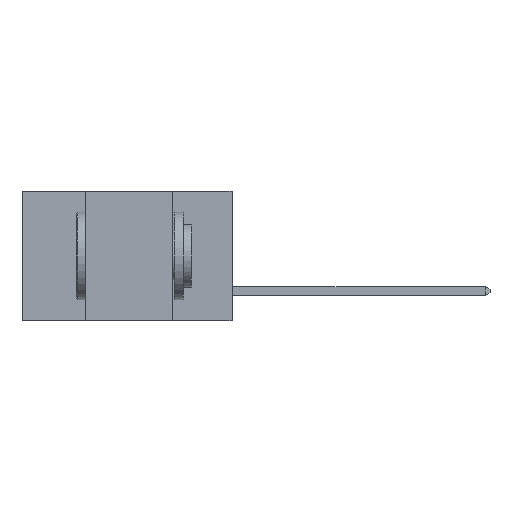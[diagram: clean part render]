
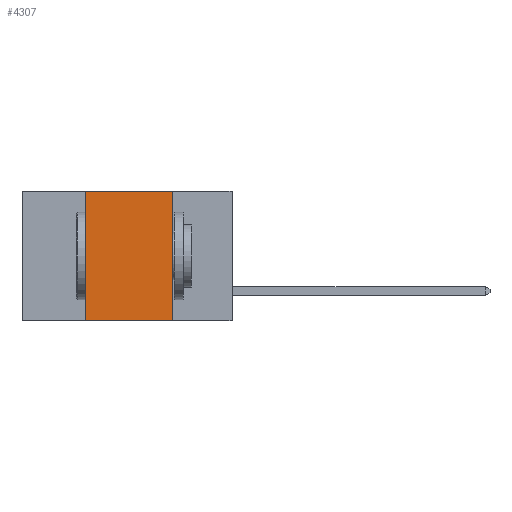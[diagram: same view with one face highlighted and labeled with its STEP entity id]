
A CAD part, left-side view. The second image highlights one B-rep face of the part: STEP entity #4307.
In plain terms, the highlighted planar face has unit normal (-1, 0, 0).
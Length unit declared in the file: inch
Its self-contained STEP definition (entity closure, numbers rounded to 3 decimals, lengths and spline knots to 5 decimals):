
#342 = EDGE_CURVE ( 'NONE', #4070, #1140, #1744, .T. ) ;
#444 = DIRECTION ( 'NONE',  ( 0., -1., 0. ) ) ;
#629 = CARTESIAN_POINT ( 'NONE',  ( 0., 0.17, 0. ) ) ;
#809 = VERTEX_POINT ( 'NONE', #4043 ) ;
#903 = VECTOR ( 'NONE', #8143, 39.37008 ) ;
#1140 = VERTEX_POINT ( 'NONE', #629 ) ;
#1716 = EDGE_LOOP ( 'NONE', ( #3507, #3320, #3019, #2835 ) ) ;
#1744 = LINE ( 'NONE', #1853, #8644 ) ;
#1853 = CARTESIAN_POINT ( 'NONE',  ( 0., 0.6, 0. ) ) ;
#2090 = CARTESIAN_POINT ( 'NONE',  ( 0., 0.17, 0. ) ) ;
#2262 = VECTOR ( 'NONE', #5062, 39.37008 ) ;
#2835 = ORIENTED_EDGE ( 'NONE', *, *, #5515, .T. ) ;
#3019 = ORIENTED_EDGE ( 'NONE', *, *, #7016, .F. ) ;
#3320 = ORIENTED_EDGE ( 'NONE', *, *, #342, .F. ) ;
#3507 = ORIENTED_EDGE ( 'NONE', *, *, #10204, .F. ) ;
#4043 = CARTESIAN_POINT ( 'NONE',  ( 0., 0.42, -0.37 ) ) ;
#4070 = VERTEX_POINT ( 'NONE', #8064 ) ;
#4307 = ADVANCED_FACE ( 'NONE', ( #5302 ), #6507, .F. ) ;
#4611 = LINE ( 'NONE', #9929, #2262 ) ;
#5062 = DIRECTION ( 'NONE',  ( 0., 0., 1. ) ) ;
#5235 = LINE ( 'NONE', #2090, #903 ) ;
#5302 = FACE_OUTER_BOUND ( 'NONE', #1716, .T. ) ;
#5407 = AXIS2_PLACEMENT_3D ( 'NONE', #6657, #6494, #6481 ) ;
#5515 = EDGE_CURVE ( 'NONE', #809, #6488, #6075, .T. ) ;
#6075 = LINE ( 'NONE', #10345, #10175 ) ;
#6481 = DIRECTION ( 'NONE',  ( 0., 0., -1. ) ) ;
#6488 = VERTEX_POINT ( 'NONE', #10112 ) ;
#6494 = DIRECTION ( 'NONE',  ( 1., 0., 0. ) ) ;
#6507 = PLANE ( 'NONE',  #5407 ) ;
#6657 = CARTESIAN_POINT ( 'NONE',  ( 0., 0.6, 0. ) ) ;
#7016 = EDGE_CURVE ( 'NONE', #809, #4070, #4611, .T. ) ;
#8064 = CARTESIAN_POINT ( 'NONE',  ( 0., 0.42, 0. ) ) ;
#8143 = DIRECTION ( 'NONE',  ( 0., 0., -1. ) ) ;
#8644 = VECTOR ( 'NONE', #10416, 39.37008 ) ;
#9929 = CARTESIAN_POINT ( 'NONE',  ( 0., 0.42, 0. ) ) ;
#10112 = CARTESIAN_POINT ( 'NONE',  ( 0., 0.17, -0.37 ) ) ;
#10175 = VECTOR ( 'NONE', #444, 39.37008 ) ;
#10204 = EDGE_CURVE ( 'NONE', #1140, #6488, #5235, .T. ) ;
#10345 = CARTESIAN_POINT ( 'NONE',  ( 0., 0.6, -0.37 ) ) ;
#10416 = DIRECTION ( 'NONE',  ( 0., -1., 0. ) ) ;
